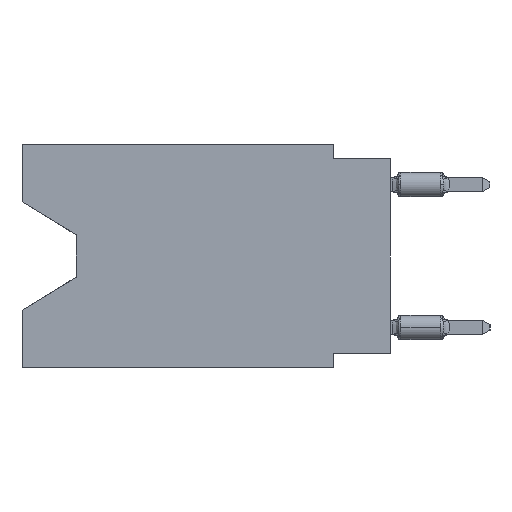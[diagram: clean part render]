
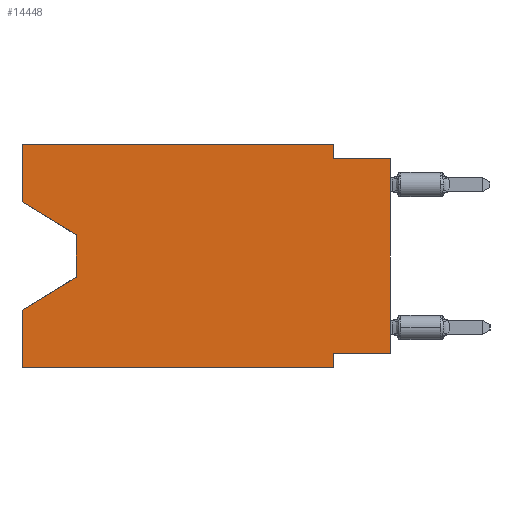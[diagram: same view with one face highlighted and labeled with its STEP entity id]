
A CAD part, left-side view. The second image highlights one B-rep face of the part: STEP entity #14448.
In plain terms, the highlighted planar face has unit normal (-1, 0, 0).
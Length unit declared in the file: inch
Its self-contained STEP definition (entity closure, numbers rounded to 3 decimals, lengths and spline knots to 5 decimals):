
#99 = EDGE_CURVE ( 'NONE', #34736, #7881, #32039, .T. ) ;
#849 = ORIENTED_EDGE ( 'NONE', *, *, #99, .T. ) ;
#1173 = CARTESIAN_POINT ( 'NONE',  ( 0., 0.645, -0.28975 ) ) ;
#1600 = CARTESIAN_POINT ( 'NONE',  ( 0., 0.1, -0.39 ) ) ;
#1628 = LINE ( 'NONE', #13455, #24278 ) ;
#1937 = CARTESIAN_POINT ( 'NONE',  ( 0., 0.645, 0. ) ) ;
#2900 = AXIS2_PLACEMENT_3D ( 'NONE', #8593, #38336, #17333 ) ;
#2912 = CARTESIAN_POINT ( 'NONE',  ( 0., 0.645, 0. ) ) ;
#3238 = EDGE_CURVE ( 'NONE', #10708, #8920, #31987, .T. ) ;
#3304 = DIRECTION ( 'NONE',  ( 0., -1., 0. ) ) ;
#3822 = VERTEX_POINT ( 'NONE', #21397 ) ;
#4136 = DIRECTION ( 'NONE',  ( 0., 0., -1. ) ) ;
#4222 = ORIENTED_EDGE ( 'NONE', *, *, #4512, .T. ) ;
#4345 = EDGE_CURVE ( 'NONE', #22701, #15219, #19580, .T. ) ;
#4392 = ORIENTED_EDGE ( 'NONE', *, *, #28451, .F. ) ;
#4512 = EDGE_CURVE ( 'NONE', #3822, #34247, #11432, .T. ) ;
#5429 = VECTOR ( 'NONE', #15060, 39.37008 ) ;
#6209 = LINE ( 'NONE', #29913, #22583 ) ;
#7180 = CARTESIAN_POINT ( 'NONE',  ( 0., 0.1, 0. ) ) ;
#7512 = CARTESIAN_POINT ( 'NONE',  ( 0., 0.1, -0.39 ) ) ;
#7561 = EDGE_CURVE ( 'NONE', #10708, #15652, #6209, .T. ) ;
#7881 = VERTEX_POINT ( 'NONE', #15425 ) ;
#8282 = CARTESIAN_POINT ( 'NONE',  ( 0., 0.55, -0.232 ) ) ;
#8401 = PLANE ( 'NONE',  #2900 ) ;
#8593 = CARTESIAN_POINT ( 'NONE',  ( 0., 0.645, 0. ) ) ;
#8705 = DIRECTION ( 'NONE',  ( 0., -0.855, -0.519 ) ) ;
#8845 = CARTESIAN_POINT ( 'NONE',  ( 0., 0.645, 0. ) ) ;
#8920 = VERTEX_POINT ( 'NONE', #1173 ) ;
#9498 = VERTEX_POINT ( 'NONE', #8282 ) ;
#10127 = ORIENTED_EDGE ( 'NONE', *, *, #11861, .F. ) ;
#10708 = VERTEX_POINT ( 'NONE', #28393 ) ;
#11432 = LINE ( 'NONE', #31847, #29864 ) ;
#11567 = EDGE_LOOP ( 'NONE', ( #4222, #15515, #35932, #13911, #11706, #10127, #27878, #849, #28094, #4392, #34330, #25003 ) ) ;
#11706 = ORIENTED_EDGE ( 'NONE', *, *, #7561, .T. ) ;
#11861 = EDGE_CURVE ( 'NONE', #25810, #15652, #16347, .T. ) ;
#11920 = CARTESIAN_POINT ( 'NONE',  ( 0., 0.55, -0.158 ) ) ;
#12011 = VECTOR ( 'NONE', #32413, 39.37008 ) ;
#13370 = CARTESIAN_POINT ( 'NONE',  ( 0., 0., 0. ) ) ;
#13455 = CARTESIAN_POINT ( 'NONE',  ( 0., 0.1, 0. ) ) ;
#13911 = ORIENTED_EDGE ( 'NONE', *, *, #3238, .F. ) ;
#14104 = VECTOR ( 'NONE', #16918, 39.37008 ) ;
#14224 = DIRECTION ( 'NONE',  ( 0., 0., -1. ) ) ;
#14448 = ADVANCED_FACE ( 'NONE', ( #35235 ), #8401, .F. ) ;
#14856 = DIRECTION ( 'NONE',  ( 0., 0., 1. ) ) ;
#15060 = DIRECTION ( 'NONE',  ( 0., 0., -1. ) ) ;
#15200 = CARTESIAN_POINT ( 'NONE',  ( 0., 0.1, -0.365 ) ) ;
#15219 = VERTEX_POINT ( 'NONE', #7180 ) ;
#15375 = VECTOR ( 'NONE', #32792, 39.37008 ) ;
#15425 = CARTESIAN_POINT ( 'NONE',  ( 0., 0., -0.025 ) ) ;
#15515 = ORIENTED_EDGE ( 'NONE', *, *, #35073, .T. ) ;
#15652 = VERTEX_POINT ( 'NONE', #7512 ) ;
#16132 = CARTESIAN_POINT ( 'NONE',  ( 0., 0.1, -0.025 ) ) ;
#16347 = LINE ( 'NONE', #1600, #30073 ) ;
#16918 = DIRECTION ( 'NONE',  ( 0., 0.855, -0.519 ) ) ;
#17317 = CARTESIAN_POINT ( 'NONE',  ( 0., 0., -0.365 ) ) ;
#17333 = DIRECTION ( 'NONE',  ( 0., 0., -1. ) ) ;
#17415 = CARTESIAN_POINT ( 'NONE',  ( 0., 0.55, -0.158 ) ) ;
#17451 = VECTOR ( 'NONE', #24691, 39.37008 ) ;
#17811 = VECTOR ( 'NONE', #24378, 39.37008 ) ;
#19580 = LINE ( 'NONE', #1937, #17451 ) ;
#19899 = DIRECTION ( 'NONE',  ( 0., -1., 0. ) ) ;
#20421 = LINE ( 'NONE', #37555, #14104 ) ;
#20547 = LINE ( 'NONE', #29302, #12011 ) ;
#21397 = CARTESIAN_POINT ( 'NONE',  ( 0., 0.645, -0.10025 ) ) ;
#22170 = EDGE_CURVE ( 'NONE', #9498, #8920, #20421, .T. ) ;
#22583 = VECTOR ( 'NONE', #3304, 39.37008 ) ;
#22701 = VERTEX_POINT ( 'NONE', #2912 ) ;
#22826 = CARTESIAN_POINT ( 'NONE',  ( 0., 0., -0.025 ) ) ;
#24278 = VECTOR ( 'NONE', #14224, 39.37008 ) ;
#24378 = DIRECTION ( 'NONE',  ( 0., 0., 1. ) ) ;
#24691 = DIRECTION ( 'NONE',  ( 0., -1., 0. ) ) ;
#25003 = ORIENTED_EDGE ( 'NONE', *, *, #37018, .F. ) ;
#25810 = VERTEX_POINT ( 'NONE', #15200 ) ;
#26558 = LINE ( 'NONE', #17415, #5429 ) ;
#27559 = VERTEX_POINT ( 'NONE', #16132 ) ;
#27652 = CARTESIAN_POINT ( 'NONE',  ( 0., 0.645, 0. ) ) ;
#27878 = ORIENTED_EDGE ( 'NONE', *, *, #31217, .F. ) ;
#28094 = ORIENTED_EDGE ( 'NONE', *, *, #35336, .F. ) ;
#28393 = CARTESIAN_POINT ( 'NONE',  ( 0., 0.645, -0.39 ) ) ;
#28451 = EDGE_CURVE ( 'NONE', #15219, #27559, #1628, .T. ) ;
#29302 = CARTESIAN_POINT ( 'NONE',  ( 0., 0., -0.365 ) ) ;
#29864 = VECTOR ( 'NONE', #8705, 39.37008 ) ;
#29913 = CARTESIAN_POINT ( 'NONE',  ( 0., 0.645, -0.39 ) ) ;
#30073 = VECTOR ( 'NONE', #4136, 39.37008 ) ;
#30581 = LINE ( 'NONE', #27652, #17811 ) ;
#31217 = EDGE_CURVE ( 'NONE', #34736, #25810, #20547, .T. ) ;
#31847 = CARTESIAN_POINT ( 'NONE',  ( 0., 0.645, -0.10025 ) ) ;
#31987 = LINE ( 'NONE', #8845, #34780 ) ;
#32039 = LINE ( 'NONE', #13370, #15375 ) ;
#32413 = DIRECTION ( 'NONE',  ( 0., 1., 0. ) ) ;
#32792 = DIRECTION ( 'NONE',  ( 0., 0., 1. ) ) ;
#34247 = VERTEX_POINT ( 'NONE', #11920 ) ;
#34330 = ORIENTED_EDGE ( 'NONE', *, *, #4345, .F. ) ;
#34736 = VERTEX_POINT ( 'NONE', #17317 ) ;
#34780 = VECTOR ( 'NONE', #14856, 39.37008 ) ;
#35073 = EDGE_CURVE ( 'NONE', #34247, #9498, #26558, .T. ) ;
#35235 = FACE_OUTER_BOUND ( 'NONE', #11567, .T. ) ;
#35336 = EDGE_CURVE ( 'NONE', #27559, #7881, #37229, .T. ) ;
#35833 = VECTOR ( 'NONE', #19899, 39.37008 ) ;
#35932 = ORIENTED_EDGE ( 'NONE', *, *, #22170, .T. ) ;
#37018 = EDGE_CURVE ( 'NONE', #3822, #22701, #30581, .T. ) ;
#37229 = LINE ( 'NONE', #22826, #35833 ) ;
#37555 = CARTESIAN_POINT ( 'NONE',  ( 0., 0.55, -0.232 ) ) ;
#38336 = DIRECTION ( 'NONE',  ( 1., 0., 0. ) ) ;
